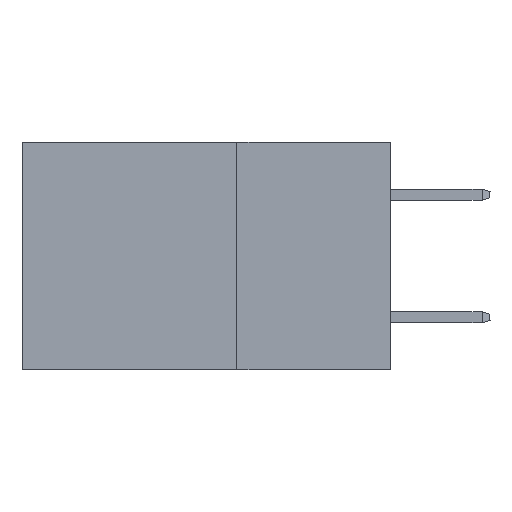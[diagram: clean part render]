
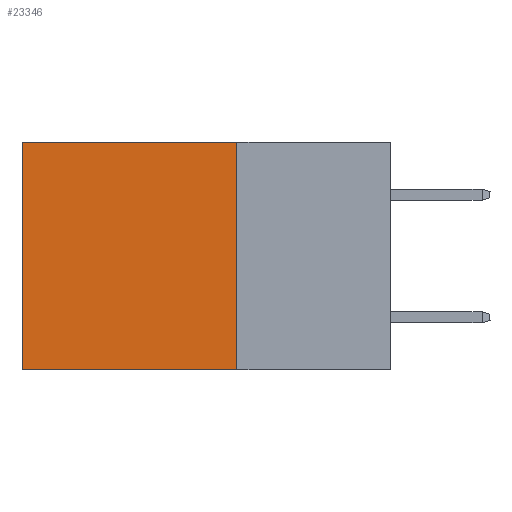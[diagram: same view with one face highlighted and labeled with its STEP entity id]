
A CAD part, left-side view. The second image highlights one B-rep face of the part: STEP entity #23346.
In plain terms, the highlighted planar face has unit normal (-1, 0, 0).
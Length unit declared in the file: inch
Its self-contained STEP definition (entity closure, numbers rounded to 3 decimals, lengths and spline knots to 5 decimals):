
#213 = LINE ( 'NONE', #33989, #30687 ) ;
#402 = EDGE_LOOP ( 'NONE', ( #38392, #4908, #27169, #7039 ) ) ;
#802 = PLANE ( 'NONE',  #16102 ) ;
#947 = VERTEX_POINT ( 'NONE', #2165 ) ;
#2165 = CARTESIAN_POINT ( 'NONE',  ( 0.2875, 0.6, -0.37 ) ) ;
#4331 = EDGE_CURVE ( 'NONE', #30868, #20619, #11871, .T. ) ;
#4908 = ORIENTED_EDGE ( 'NONE', *, *, #5281, .F. ) ;
#4931 = CARTESIAN_POINT ( 'NONE',  ( 0.2875, 0.25, -0.37 ) ) ;
#5281 = EDGE_CURVE ( 'NONE', #20619, #947, #18551, .T. ) ;
#5355 = DIRECTION ( 'NONE',  ( 0., 1., 0. ) ) ;
#7039 = ORIENTED_EDGE ( 'NONE', *, *, #18652, .T. ) ;
#7647 = VECTOR ( 'NONE', #39885, 39.37008 ) ;
#9159 = FACE_OUTER_BOUND ( 'NONE', #402, .T. ) ;
#9626 = DIRECTION ( 'NONE',  ( 0., 0., -1. ) ) ;
#11871 = LINE ( 'NONE', #22534, #37132 ) ;
#12094 = VECTOR ( 'NONE', #5355, 39.37008 ) ;
#12895 = CARTESIAN_POINT ( 'NONE',  ( 0.2875, 0.6, 0. ) ) ;
#13913 = DIRECTION ( 'NONE',  ( 0., 0., -1. ) ) ;
#15041 = CARTESIAN_POINT ( 'NONE',  ( 0.2875, 0.25, 0. ) ) ;
#16102 = AXIS2_PLACEMENT_3D ( 'NONE', #33670, #23873, #13913 ) ;
#18551 = LINE ( 'NONE', #26635, #7647 ) ;
#18652 = EDGE_CURVE ( 'NONE', #30868, #24367, #40485, .T. ) ;
#20611 = DIRECTION ( 'NONE',  ( 0., 0., -1. ) ) ;
#20619 = VERTEX_POINT ( 'NONE', #4931 ) ;
#22534 = CARTESIAN_POINT ( 'NONE',  ( 0.2875, 0.25, 0. ) ) ;
#23346 = ADVANCED_FACE ( 'NONE', ( #9159 ), #802, .F. ) ;
#23873 = DIRECTION ( 'NONE',  ( 1., 0., 0. ) ) ;
#24367 = VERTEX_POINT ( 'NONE', #12895 ) ;
#26635 = CARTESIAN_POINT ( 'NONE',  ( 0.2875, 0.25, -0.37 ) ) ;
#27123 = EDGE_CURVE ( 'NONE', #24367, #947, #213, .T. ) ;
#27169 = ORIENTED_EDGE ( 'NONE', *, *, #4331, .F. ) ;
#30687 = VECTOR ( 'NONE', #20611, 39.37008 ) ;
#30868 = VERTEX_POINT ( 'NONE', #32355 ) ;
#32355 = CARTESIAN_POINT ( 'NONE',  ( 0.2875, 0.25, 0. ) ) ;
#33670 = CARTESIAN_POINT ( 'NONE',  ( 0.2875, 0.25, 0. ) ) ;
#33989 = CARTESIAN_POINT ( 'NONE',  ( 0.2875, 0.6, 0. ) ) ;
#37132 = VECTOR ( 'NONE', #9626, 39.37008 ) ;
#38392 = ORIENTED_EDGE ( 'NONE', *, *, #27123, .T. ) ;
#39885 = DIRECTION ( 'NONE',  ( 0., 1., 0. ) ) ;
#40485 = LINE ( 'NONE', #15041, #12094 ) ;
